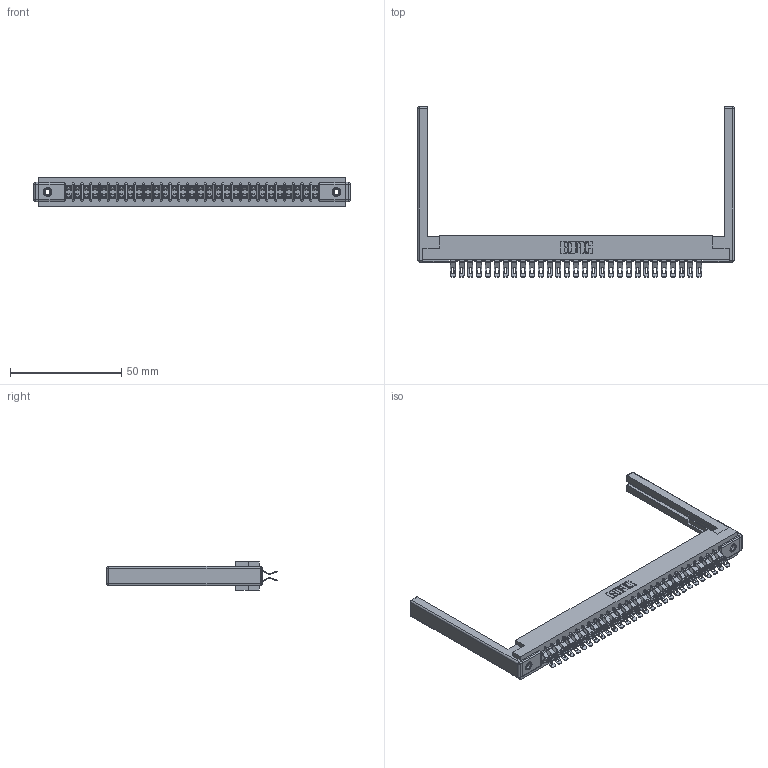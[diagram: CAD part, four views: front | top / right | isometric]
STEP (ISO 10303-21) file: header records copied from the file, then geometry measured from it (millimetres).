
FILE_DESCRIPTION (( 'STEP AP203' ), '1' );
FILE_NAME ('307-058-455-268.STEP', '2020-09-30T12:43:09', ( '' ), ( '' ), 'SwSTEP 2.0', 'SolidWorks 2020', '' );
FILE_SCHEMA (( 'CONFIG_CONTROL_DESIGN' ));
Length unit declared in the file: inch
Products named in the file (5): 307-290-001_555; 307-058-455-268; 307-220-068; 307 Part_.156 Dia Mounting Holes; 345-250-001_345-250-001-102
Assembly tree (63 placements, depth 2):
  307-058-455-268
    307 Part_.156 Dia Mounting Holes
    307-290-001_555  x58
    307-220-068  x2
    345-250-001_345-250-001-102  x2
Bounding box: 142.34 x 76.71 x 12.7 mm (x, y, z)
Volume: 19597.6 mm3; surface area: 23297.6 mm2
Topology: 63 solids, 63 shells, 3840 faces, 11211 edges, 7294 vertices
Faces by surface type: plane 2130, cylinder 1626, sphere 68, cone 12, torus 4
Entity records: 30688 total; most frequent: CARTESIAN_POINT 5006, ORIENTED_EDGE 4954, DIRECTION 4931, EDGE_CURVE 2477, VECTOR 1881, LINE 1881, VERTEX_POINT 1600, AXIS2_PLACEMENT_3D 1525
